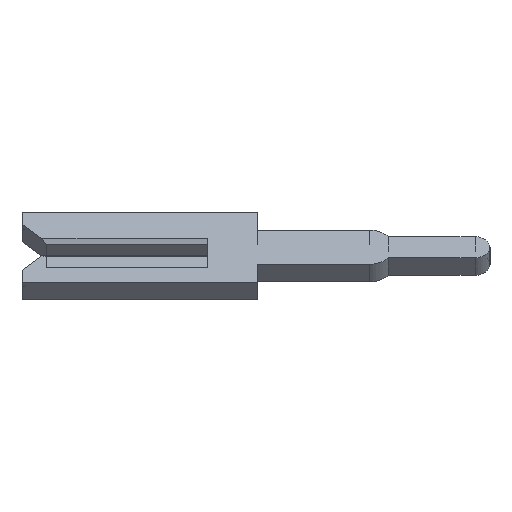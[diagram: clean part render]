
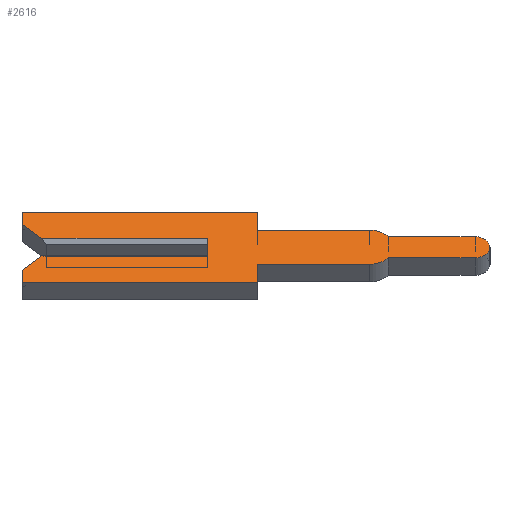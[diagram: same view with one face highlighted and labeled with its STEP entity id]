
A CAD part, left-side view. The second image highlights one B-rep face of the part: STEP entity #2616.
In plain terms, the highlighted face is planar.
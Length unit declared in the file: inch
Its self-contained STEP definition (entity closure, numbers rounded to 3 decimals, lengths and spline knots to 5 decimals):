
#50 = ORIENTED_EDGE ( 'NONE', *, *, #1258, .F. ) ;
#77 = ORIENTED_EDGE ( 'NONE', *, *, #1814, .F. ) ;
#81 = VERTEX_POINT ( 'NONE', #1898 ) ;
#86 = VECTOR ( 'NONE', #1461, 39.37008 ) ;
#99 = ORIENTED_EDGE ( 'NONE', *, *, #1094, .F. ) ;
#109 = VECTOR ( 'NONE', #1141, 39.37008 ) ;
#144 = LINE ( 'NONE', #1497, #1853 ) ;
#145 = CIRCLE ( 'NONE', #1811, 0.012 ) ;
#162 = DIRECTION ( 'NONE',  ( 0., -1., 0. ) ) ;
#168 = ORIENTED_EDGE ( 'NONE', *, *, #2783, .F. ) ;
#169 = AXIS2_PLACEMENT_3D ( 'NONE', #667, #473, #2036 ) ;
#176 = CARTESIAN_POINT ( 'NONE',  ( -0.01, -0.216, -0.012 ) ) ;
#220 = CARTESIAN_POINT ( 'NONE',  ( -0.01, 0.15, 0.01 ) ) ;
#269 = EDGE_CURVE ( 'NONE', #2452, #81, #2631, .T. ) ;
#282 = EDGE_CURVE ( 'NONE', #1863, #2430, #2398, .T. ) ;
#306 = LINE ( 'NONE', #1315, #2540 ) ;
#318 = VERTEX_POINT ( 'NONE', #358 ) ;
#324 = VECTOR ( 'NONE', #806, 39.37008 ) ;
#346 = VECTOR ( 'NONE', #1296, 39.37008 ) ;
#358 = CARTESIAN_POINT ( 'NONE',  ( -0.01, -0.1305, 0.0195 ) ) ;
#375 = CARTESIAN_POINT ( 'NONE',  ( -0.01, 0.15, -0.04 ) ) ;
#383 = VECTOR ( 'NONE', #401, 39.37008 ) ;
#401 = DIRECTION ( 'NONE',  ( 0., 1., 0. ) ) ;
#443 = VERTEX_POINT ( 'NONE', #596 ) ;
#461 = DIRECTION ( 'NONE',  ( 0., 0., -1. ) ) ;
#469 = CARTESIAN_POINT ( 'NONE',  ( -0.01, 0.15, 0.04 ) ) ;
#473 = DIRECTION ( 'NONE',  ( 1., 0., 0. ) ) ;
#479 = LINE ( 'NONE', #2015, #2109 ) ;
#520 = VECTOR ( 'NONE', #2665, 39.37008 ) ;
#536 = ORIENTED_EDGE ( 'NONE', *, *, #2600, .T. ) ;
#553 = VECTOR ( 'NONE', #1036, 39.37008 ) ;
#555 = LINE ( 'NONE', #717, #725 ) ;
#596 = CARTESIAN_POINT ( 'NONE',  ( -0.01, 0.134, 0.01 ) ) ;
#609 = DIRECTION ( 'NONE',  ( 1., 0., 0. ) ) ;
#639 = DIRECTION ( 'NONE',  ( 0., 0., -1. ) ) ;
#648 = ORIENTED_EDGE ( 'NONE', *, *, #2261, .F. ) ;
#661 = AXIS2_PLACEMENT_3D ( 'NONE', #1995, #609, #2672 ) ;
#667 = CARTESIAN_POINT ( 'NONE',  ( -0.01, -0.1305, 0. ) ) ;
#682 = VERTEX_POINT ( 'NONE', #848 ) ;
#688 = CARTESIAN_POINT ( 'NONE',  ( -0.01, -0.14587, -0.012 ) ) ;
#690 = LINE ( 'NONE', #220, #109 ) ;
#717 = CARTESIAN_POINT ( 'NONE',  ( -0.01, -0.1305, 0.012 ) ) ;
#721 = LINE ( 'NONE', #788, #553 ) ;
#725 = VECTOR ( 'NONE', #2813, 39.37008 ) ;
#747 = VERTEX_POINT ( 'NONE', #2723 ) ;
#750 = EDGE_CURVE ( 'NONE', #318, #2844, #2854, .T. ) ;
#788 = CARTESIAN_POINT ( 'NONE',  ( -0.01, 0., 0.0065 ) ) ;
#806 = DIRECTION ( 'NONE',  ( 0., 0., 1. ) ) ;
#827 = CARTESIAN_POINT ( 'NONE',  ( -0.01, 0.15, -0.026 ) ) ;
#830 = VERTEX_POINT ( 'NONE', #2504 ) ;
#848 = CARTESIAN_POINT ( 'NONE',  ( -0.01, 0., 0.01 ) ) ;
#854 = EDGE_CURVE ( 'NONE', #2743, #2413, #2332, .T. ) ;
#855 = EDGE_CURVE ( 'NONE', #2271, #2196, #145, .T. ) ;
#887 = DIRECTION ( 'NONE',  ( 0., 0., 1. ) ) ;
#905 = PLANE ( 'NONE',  #169 ) ;
#910 = CARTESIAN_POINT ( 'NONE',  ( -0.01, -0.1305, 0. ) ) ;
#965 = ORIENTED_EDGE ( 'NONE', *, *, #1906, .F. ) ;
#993 = EDGE_CURVE ( 'NONE', #443, #747, #2852, .T. ) ;
#995 = VERTEX_POINT ( 'NONE', #1972 ) ;
#1003 = VECTOR ( 'NONE', #1711, 39.37008 ) ;
#1034 = ORIENTED_EDGE ( 'NONE', *, *, #282, .F. ) ;
#1036 = DIRECTION ( 'NONE',  ( 0., 0., 1. ) ) ;
#1059 = ORIENTED_EDGE ( 'NONE', *, *, #855, .F. ) ;
#1076 = CARTESIAN_POINT ( 'NONE',  ( -0.01, -0.04, -0.0195 ) ) ;
#1094 = EDGE_CURVE ( 'NONE', #1220, #2452, #2401, .T. ) ;
#1141 = DIRECTION ( 'NONE',  ( 0., -1., 0. ) ) ;
#1159 = DIRECTION ( 'NONE',  ( 0., 1., 0. ) ) ;
#1188 = ORIENTED_EDGE ( 'NONE', *, *, #1944, .F. ) ;
#1220 = VERTEX_POINT ( 'NONE', #2529 ) ;
#1232 = CARTESIAN_POINT ( 'NONE',  ( -0.01, 0.134, -0.01 ) ) ;
#1248 = DIRECTION ( 'NONE',  ( 0., -0.707, 0.707 ) ) ;
#1258 = EDGE_CURVE ( 'NONE', #2844, #2271, #555, .T. ) ;
#1284 = DIRECTION ( 'NONE',  ( 0., 0., -1. ) ) ;
#1292 = CARTESIAN_POINT ( 'NONE',  ( -0.01, -0.216, 0.012 ) ) ;
#1296 = DIRECTION ( 'NONE',  ( 0., 0.707, 0.707 ) ) ;
#1304 = ORIENTED_EDGE ( 'NONE', *, *, #1738, .F. ) ;
#1315 = CARTESIAN_POINT ( 'NONE',  ( -0.01, -0.04, 0.04 ) ) ;
#1319 = LINE ( 'NONE', #375, #2075 ) ;
#1321 = VECTOR ( 'NONE', #1159, 39.37008 ) ;
#1455 = CARTESIAN_POINT ( 'NONE',  ( -0.01, 0.1305, -0.0065 ) ) ;
#1461 = DIRECTION ( 'NONE',  ( 0., 0., -1. ) ) ;
#1472 = AXIS2_PLACEMENT_3D ( 'NONE', #910, #1585, #1284 ) ;
#1497 = CARTESIAN_POINT ( 'NONE',  ( -0.01, -0.04, 0.0195 ) ) ;
#1531 = VECTOR ( 'NONE', #1248, 39.37008 ) ;
#1548 = LINE ( 'NONE', #2463, #383 ) ;
#1556 = EDGE_LOOP ( 'NONE', ( #648, #2677, #1059, #50, #2054, #965, #2049, #1746, #168, #1679, #536, #1699, #1304, #1188, #1034, #77, #2037, #99 ) ) ;
#1569 = CARTESIAN_POINT ( 'NONE',  ( -0.01, 0.15, 0.04 ) ) ;
#1585 = DIRECTION ( 'NONE',  ( 1., 0., 0. ) ) ;
#1679 = ORIENTED_EDGE ( 'NONE', *, *, #993, .F. ) ;
#1699 = ORIENTED_EDGE ( 'NONE', *, *, #1848, .F. ) ;
#1711 = DIRECTION ( 'NONE',  ( 0., -1., 0. ) ) ;
#1738 = EDGE_CURVE ( 'NONE', #2177, #995, #2470, .T. ) ;
#1746 = ORIENTED_EDGE ( 'NONE', *, *, #854, .F. ) ;
#1748 = CARTESIAN_POINT ( 'NONE',  ( -0.01, 0.15, -0.026 ) ) ;
#1811 = AXIS2_PLACEMENT_3D ( 'NONE', #2034, #2268, #461 ) ;
#1814 = EDGE_CURVE ( 'NONE', #81, #1863, #1319, .T. ) ;
#1848 = EDGE_CURVE ( 'NONE', #995, #682, #721, .T. ) ;
#1853 = VECTOR ( 'NONE', #162, 39.37008 ) ;
#1863 = VERTEX_POINT ( 'NONE', #2412 ) ;
#1898 = CARTESIAN_POINT ( 'NONE',  ( -0.01, -0.04, -0.04 ) ) ;
#1906 = EDGE_CURVE ( 'NONE', #830, #318, #144, .T. ) ;
#1923 = DIRECTION ( 'NONE',  ( 0., 1., 0. ) ) ;
#1944 = EDGE_CURVE ( 'NONE', #2430, #2177, #1964, .T. ) ;
#1964 = LINE ( 'NONE', #1455, #1531 ) ;
#1972 = CARTESIAN_POINT ( 'NONE',  ( -0.01, 0., -0.01 ) ) ;
#1995 = CARTESIAN_POINT ( 'NONE',  ( -0.01, -0.1305, 0. ) ) ;
#2015 = CARTESIAN_POINT ( 'NONE',  ( -0.01, 0.15, 0.026 ) ) ;
#2034 = CARTESIAN_POINT ( 'NONE',  ( -0.01, -0.216, 0. ) ) ;
#2036 = DIRECTION ( 'NONE',  ( 0., 0., -1. ) ) ;
#2037 = ORIENTED_EDGE ( 'NONE', *, *, #269, .F. ) ;
#2049 = ORIENTED_EDGE ( 'NONE', *, *, #2185, .F. ) ;
#2054 = ORIENTED_EDGE ( 'NONE', *, *, #750, .F. ) ;
#2070 = CARTESIAN_POINT ( 'NONE',  ( -0.01, -0.04, -0.0195 ) ) ;
#2075 = VECTOR ( 'NONE', #1923, 39.37008 ) ;
#2104 = EDGE_CURVE ( 'NONE', #2196, #2499, #1548, .T. ) ;
#2109 = VECTOR ( 'NONE', #887, 39.37008 ) ;
#2177 = VERTEX_POINT ( 'NONE', #1232 ) ;
#2185 = EDGE_CURVE ( 'NONE', #2413, #830, #306, .T. ) ;
#2196 = VERTEX_POINT ( 'NONE', #176 ) ;
#2214 = CARTESIAN_POINT ( 'NONE',  ( -0.01, 0.1305, 0.0065 ) ) ;
#2261 = EDGE_CURVE ( 'NONE', #2499, #1220, #2718, .T. ) ;
#2268 = DIRECTION ( 'NONE',  ( 1., 0., 0. ) ) ;
#2271 = VERTEX_POINT ( 'NONE', #1292 ) ;
#2332 = LINE ( 'NONE', #469, #520 ) ;
#2398 = LINE ( 'NONE', #827, #324 ) ;
#2401 = LINE ( 'NONE', #2070, #1321 ) ;
#2402 = CARTESIAN_POINT ( 'NONE',  ( -0.01, -0.1305, -0.01 ) ) ;
#2412 = CARTESIAN_POINT ( 'NONE',  ( -0.01, 0.15, -0.04 ) ) ;
#2413 = VERTEX_POINT ( 'NONE', #2660 ) ;
#2430 = VERTEX_POINT ( 'NONE', #1748 ) ;
#2452 = VERTEX_POINT ( 'NONE', #1076 ) ;
#2463 = CARTESIAN_POINT ( 'NONE',  ( -0.01, -0.1305, -0.012 ) ) ;
#2470 = LINE ( 'NONE', #2402, #1003 ) ;
#2499 = VERTEX_POINT ( 'NONE', #688 ) ;
#2504 = CARTESIAN_POINT ( 'NONE',  ( -0.01, -0.04, 0.0195 ) ) ;
#2529 = CARTESIAN_POINT ( 'NONE',  ( -0.01, -0.1305, -0.0195 ) ) ;
#2540 = VECTOR ( 'NONE', #639, 39.37008 ) ;
#2600 = EDGE_CURVE ( 'NONE', #443, #682, #690, .T. ) ;
#2616 = ADVANCED_FACE ( 'NONE', ( #2818 ), #905, .F. ) ;
#2631 = LINE ( 'NONE', #2823, #86 ) ;
#2660 = CARTESIAN_POINT ( 'NONE',  ( -0.01, -0.04, 0.04 ) ) ;
#2665 = DIRECTION ( 'NONE',  ( 0., -1., 0. ) ) ;
#2672 = DIRECTION ( 'NONE',  ( 0., 0., -1. ) ) ;
#2677 = ORIENTED_EDGE ( 'NONE', *, *, #2104, .F. ) ;
#2706 = CARTESIAN_POINT ( 'NONE',  ( -0.01, -0.14587, 0.012 ) ) ;
#2718 = CIRCLE ( 'NONE', #661, 0.0195 ) ;
#2723 = CARTESIAN_POINT ( 'NONE',  ( -0.01, 0.15, 0.026 ) ) ;
#2743 = VERTEX_POINT ( 'NONE', #1569 ) ;
#2783 = EDGE_CURVE ( 'NONE', #747, #2743, #479, .T. ) ;
#2813 = DIRECTION ( 'NONE',  ( 0., -1., 0. ) ) ;
#2818 = FACE_OUTER_BOUND ( 'NONE', #1556, .T. ) ;
#2823 = CARTESIAN_POINT ( 'NONE',  ( -0.01, -0.04, -0.04 ) ) ;
#2844 = VERTEX_POINT ( 'NONE', #2706 ) ;
#2852 = LINE ( 'NONE', #2214, #346 ) ;
#2854 = CIRCLE ( 'NONE', #1472, 0.0195 ) ;
